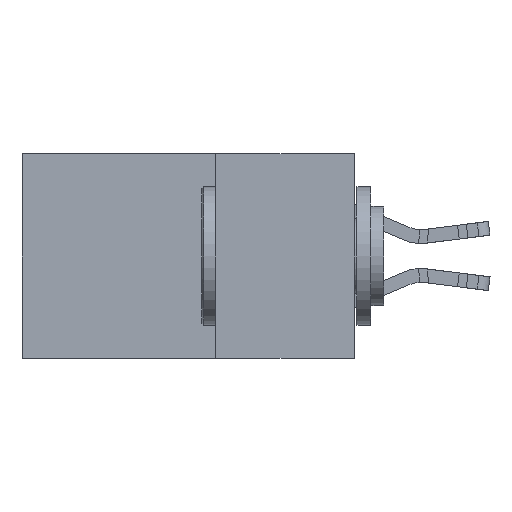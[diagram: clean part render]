
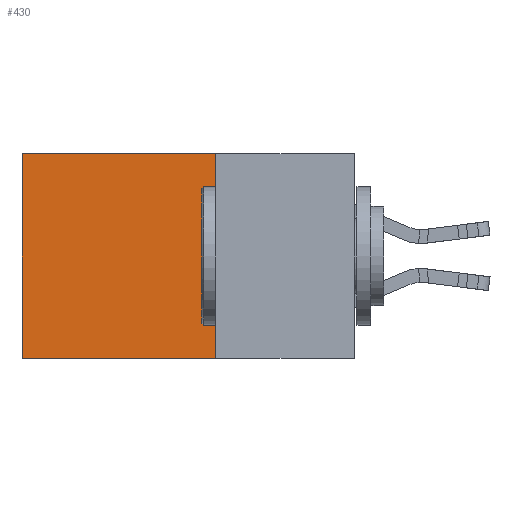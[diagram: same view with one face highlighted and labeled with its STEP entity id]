
A CAD part, left-side view. The second image highlights one B-rep face of the part: STEP entity #430.
In plain terms, the highlighted planar face has unit normal (-1, 0, 0).
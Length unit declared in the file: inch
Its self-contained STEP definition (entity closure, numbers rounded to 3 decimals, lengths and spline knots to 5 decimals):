
#430 = ADVANCED_FACE ( 'NONE', ( #21451 ), #5653, .F. ) ;
#1405 = VERTEX_POINT ( 'NONE', #4827 ) ;
#1427 = DIRECTION ( 'NONE',  ( 1., 0., 0. ) ) ;
#1448 = ORIENTED_EDGE ( 'NONE', *, *, #24595, .F. ) ;
#1463 = ORIENTED_EDGE ( 'NONE', *, *, #11764, .F. ) ;
#2571 = CARTESIAN_POINT ( 'NONE',  ( 0.2615, 0.25, 0. ) ) ;
#3811 = EDGE_CURVE ( 'NONE', #24820, #8299, #17454, .T. ) ;
#4827 = CARTESIAN_POINT ( 'NONE',  ( 0.2615, 0.25, -0.37 ) ) ;
#4980 = DIRECTION ( 'NONE',  ( 0., 0., -1. ) ) ;
#5389 = CARTESIAN_POINT ( 'NONE',  ( 0.2615, 0.6, -0.37 ) ) ;
#5653 = PLANE ( 'NONE',  #23084 ) ;
#6294 = CARTESIAN_POINT ( 'NONE',  ( 0.2615, 0.25, -0.37 ) ) ;
#8299 = VERTEX_POINT ( 'NONE', #9948 ) ;
#9948 = CARTESIAN_POINT ( 'NONE',  ( 0.2615, 0.6, 0. ) ) ;
#11764 = EDGE_CURVE ( 'NONE', #1405, #14165, #13984, .T. ) ;
#12111 = DIRECTION ( 'NONE',  ( 0., 0., -1. ) ) ;
#12231 = EDGE_LOOP ( 'NONE', ( #18667, #1463, #1448, #17093 ) ) ;
#13094 = LINE ( 'NONE', #16133, #22953 ) ;
#13984 = LINE ( 'NONE', #16981, #19277 ) ;
#14121 = VECTOR ( 'NONE', #4980, 39.37008 ) ;
#14165 = VERTEX_POINT ( 'NONE', #5389 ) ;
#15157 = CARTESIAN_POINT ( 'NONE',  ( 0.2615, 0.6, -0.37 ) ) ;
#16133 = CARTESIAN_POINT ( 'NONE',  ( 0.2615, 0.25, -0.37 ) ) ;
#16981 = CARTESIAN_POINT ( 'NONE',  ( 0.2615, 0.25, -0.37 ) ) ;
#17093 = ORIENTED_EDGE ( 'NONE', *, *, #3811, .T. ) ;
#17454 = LINE ( 'NONE', #2571, #22670 ) ;
#18134 = DIRECTION ( 'NONE',  ( 0., 0., -1. ) ) ;
#18667 = ORIENTED_EDGE ( 'NONE', *, *, #23066, .T. ) ;
#18738 = CARTESIAN_POINT ( 'NONE',  ( 0.2615, 0.25, 0. ) ) ;
#18998 = DIRECTION ( 'NONE',  ( 0., 1., 0. ) ) ;
#19277 = VECTOR ( 'NONE', #18998, 39.37008 ) ;
#19408 = LINE ( 'NONE', #15157, #14121 ) ;
#21451 = FACE_OUTER_BOUND ( 'NONE', #12231, .T. ) ;
#22670 = VECTOR ( 'NONE', #25788, 39.37008 ) ;
#22953 = VECTOR ( 'NONE', #18134, 39.37008 ) ;
#23066 = EDGE_CURVE ( 'NONE', #8299, #14165, #19408, .T. ) ;
#23084 = AXIS2_PLACEMENT_3D ( 'NONE', #6294, #1427, #12111 ) ;
#24595 = EDGE_CURVE ( 'NONE', #24820, #1405, #13094, .T. ) ;
#24820 = VERTEX_POINT ( 'NONE', #18738 ) ;
#25788 = DIRECTION ( 'NONE',  ( 0., 1., 0. ) ) ;
